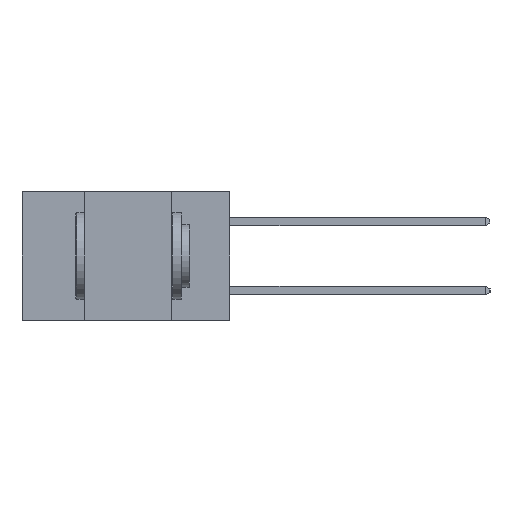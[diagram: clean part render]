
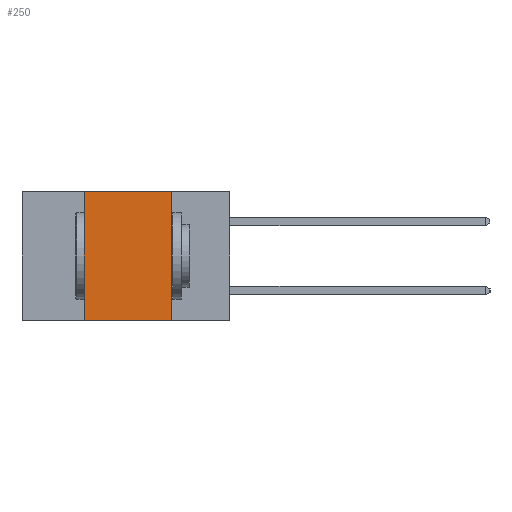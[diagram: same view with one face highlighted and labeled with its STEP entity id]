
A CAD part, left-side view. The second image highlights one B-rep face of the part: STEP entity #250.
In plain terms, the highlighted planar face has unit normal (-1, 0, 0).
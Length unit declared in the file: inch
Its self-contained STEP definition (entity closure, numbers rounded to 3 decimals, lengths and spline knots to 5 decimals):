
#168 = ORIENTED_EDGE ( 'NONE', *, *, #15943, .T. ) ;
#250 = ADVANCED_FACE ( 'NONE', ( #16926 ), #9900, .F. ) ;
#544 = DIRECTION ( 'NONE',  ( 1., 0., 0. ) ) ;
#2018 = ORIENTED_EDGE ( 'NONE', *, *, #7956, .F. ) ;
#2052 = DIRECTION ( 'NONE',  ( 0., 0., -1. ) ) ;
#2393 = CARTESIAN_POINT ( 'NONE',  ( 0., 0.6, 0. ) ) ;
#2661 = ORIENTED_EDGE ( 'NONE', *, *, #12512, .F. ) ;
#2861 = VECTOR ( 'NONE', #2052, 39.37008 ) ;
#2908 = CARTESIAN_POINT ( 'NONE',  ( 0., 0.42, 0. ) ) ;
#2986 = VERTEX_POINT ( 'NONE', #2908 ) ;
#3033 = CARTESIAN_POINT ( 'NONE',  ( 0., 0.17, 0. ) ) ;
#3665 = LINE ( 'NONE', #9388, #10438 ) ;
#4136 = VERTEX_POINT ( 'NONE', #3033 ) ;
#4549 = AXIS2_PLACEMENT_3D ( 'NONE', #2393, #544, #6618 ) ;
#6292 = VECTOR ( 'NONE', #8547, 39.37008 ) ;
#6568 = LINE ( 'NONE', #14357, #2861 ) ;
#6618 = DIRECTION ( 'NONE',  ( 0., 0., -1. ) ) ;
#7956 = EDGE_CURVE ( 'NONE', #4136, #10183, #6568, .T. ) ;
#7977 = CARTESIAN_POINT ( 'NONE',  ( 0., 0.6, 0. ) ) ;
#8547 = DIRECTION ( 'NONE',  ( 0., 0., 1. ) ) ;
#9388 = CARTESIAN_POINT ( 'NONE',  ( 0., 0.6, -0.37 ) ) ;
#9900 = PLANE ( 'NONE',  #4549 ) ;
#10183 = VERTEX_POINT ( 'NONE', #12807 ) ;
#10438 = VECTOR ( 'NONE', #17581, 39.37008 ) ;
#10685 = EDGE_LOOP ( 'NONE', ( #2018, #2661, #13809, #168 ) ) ;
#11694 = LINE ( 'NONE', #7977, #14941 ) ;
#12512 = EDGE_CURVE ( 'NONE', #2986, #4136, #11694, .T. ) ;
#12807 = CARTESIAN_POINT ( 'NONE',  ( 0., 0.17, -0.37 ) ) ;
#13809 = ORIENTED_EDGE ( 'NONE', *, *, #14682, .F. ) ;
#14357 = CARTESIAN_POINT ( 'NONE',  ( 0., 0.17, -0.37 ) ) ;
#14682 = EDGE_CURVE ( 'NONE', #16215, #2986, #16731, .T. ) ;
#14941 = VECTOR ( 'NONE', #16143, 39.37008 ) ;
#15347 = CARTESIAN_POINT ( 'NONE',  ( 0., 0.42, -0.37 ) ) ;
#15943 = EDGE_CURVE ( 'NONE', #16215, #10183, #3665, .T. ) ;
#16143 = DIRECTION ( 'NONE',  ( 0., -1., 0. ) ) ;
#16215 = VERTEX_POINT ( 'NONE', #17145 ) ;
#16731 = LINE ( 'NONE', #15347, #6292 ) ;
#16926 = FACE_OUTER_BOUND ( 'NONE', #10685, .T. ) ;
#17145 = CARTESIAN_POINT ( 'NONE',  ( 0., 0.42, -0.37 ) ) ;
#17581 = DIRECTION ( 'NONE',  ( 0., -1., 0. ) ) ;
